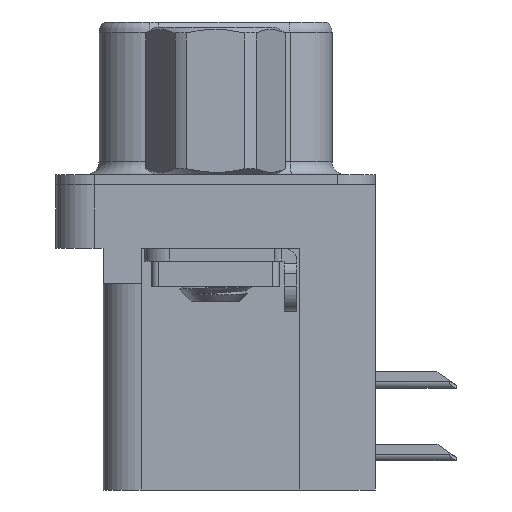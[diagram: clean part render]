
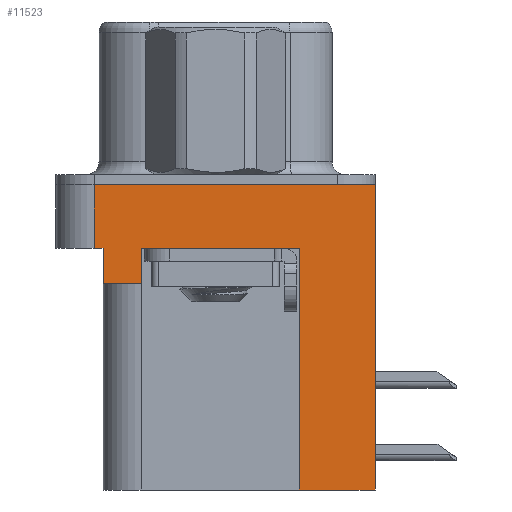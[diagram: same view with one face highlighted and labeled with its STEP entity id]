
A CAD part, left-side view. The second image highlights one B-rep face of the part: STEP entity #11523.
In plain terms, the highlighted planar face has unit normal (-1, 0, 0).
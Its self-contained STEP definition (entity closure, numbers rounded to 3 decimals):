
#674 = CARTESIAN_POINT ( 'NONE',  ( -2.91, -6.275, -2.5 ) ) ;
#1335 = VERTEX_POINT ( 'NONE', #20041 ) ;
#1969 = VECTOR ( 'NONE', #5061, 1000. ) ;
#2468 = VERTEX_POINT ( 'NONE', #5001 ) ;
#3280 = CARTESIAN_POINT ( 'NONE',  ( -2.91, -3.295, -12. ) ) ;
#3529 = VECTOR ( 'NONE', #9957, 1000. ) ;
#3999 = DIRECTION ( 'NONE',  ( 0., 1., 0. ) ) ;
#4079 = ORIENTED_EDGE ( 'NONE', *, *, #15151, .F. ) ;
#4685 = ORIENTED_EDGE ( 'NONE', *, *, #15433, .T. ) ;
#4845 = CARTESIAN_POINT ( 'NONE',  ( -2.91, 4.775, -2.5 ) ) ;
#4913 = DIRECTION ( 'NONE',  ( 0., 0., 1. ) ) ;
#4947 = ORIENTED_EDGE ( 'NONE', *, *, #13499, .T. ) ;
#5001 = CARTESIAN_POINT ( 'NONE',  ( -2.91, 4.425, -2.5 ) ) ;
#5061 = DIRECTION ( 'NONE',  ( 0., 0., 1. ) ) ;
#5863 = LINE ( 'NONE', #9686, #18467 ) ;
#6072 = VERTEX_POINT ( 'NONE', #17109 ) ;
#6803 = DIRECTION ( 'NONE',  ( 0., 1., 0. ) ) ;
#6964 = VECTOR ( 'NONE', #4913, 1000. ) ;
#7417 = ORIENTED_EDGE ( 'NONE', *, *, #13895, .T. ) ;
#7505 = VECTOR ( 'NONE', #6803, 1000. ) ;
#7864 = VERTEX_POINT ( 'NONE', #14182 ) ;
#8044 = LINE ( 'NONE', #17987, #3529 ) ;
#8852 = LINE ( 'NONE', #14051, #17487 ) ;
#9097 = VERTEX_POINT ( 'NONE', #12166 ) ;
#9280 = ORIENTED_EDGE ( 'NONE', *, *, #15211, .F. ) ;
#9686 = CARTESIAN_POINT ( 'NONE',  ( -2.91, 2.895, -3.9 ) ) ;
#9844 = CARTESIAN_POINT ( 'NONE',  ( -2.91, 4.775, 0. ) ) ;
#9957 = DIRECTION ( 'NONE',  ( 0., -1., 0. ) ) ;
#10002 = ORIENTED_EDGE ( 'NONE', *, *, #15378, .F. ) ;
#10162 = LINE ( 'NONE', #674, #11233 ) ;
#10411 = ORIENTED_EDGE ( 'NONE', *, *, #15206, .F. ) ;
#10449 = LINE ( 'NONE', #13562, #1969 ) ;
#11233 = VECTOR ( 'NONE', #12330, 1000. ) ;
#11523 = ADVANCED_FACE ( 'NONE', ( #19869 ), #17923, .T. ) ;
#11582 = DIRECTION ( 'NONE',  ( 0., 0., 1. ) ) ;
#11702 = DIRECTION ( 'NONE',  ( 0., 0., 1. ) ) ;
#11998 = LINE ( 'NONE', #4845, #16191 ) ;
#12139 = CARTESIAN_POINT ( 'NONE',  ( -2.91, -6.275, -12. ) ) ;
#12166 = CARTESIAN_POINT ( 'NONE',  ( -2.91, 2.895, -2.5 ) ) ;
#12330 = DIRECTION ( 'NONE',  ( 0., -1., 0. ) ) ;
#12501 = LINE ( 'NONE', #3280, #6964 ) ;
#12734 = CARTESIAN_POINT ( 'NONE',  ( -2.91, 4.425, -3.9 ) ) ;
#13024 = DIRECTION ( 'NONE',  ( 0., 0., 1. ) ) ;
#13079 = DIRECTION ( 'NONE',  ( 0., -1., 0. ) ) ;
#13087 = CARTESIAN_POINT ( 'NONE',  ( -2.91, -3.295, -12. ) ) ;
#13499 = EDGE_CURVE ( 'NONE', #9097, #1335, #10162, .T. ) ;
#13529 = VECTOR ( 'NONE', #13079, 1000. ) ;
#13562 = CARTESIAN_POINT ( 'NONE',  ( -2.91, -6.275, -2.5 ) ) ;
#13895 = EDGE_CURVE ( 'NONE', #6072, #9097, #5863, .T. ) ;
#14051 = CARTESIAN_POINT ( 'NONE',  ( -2.91, 4.425, -3.9 ) ) ;
#14182 = CARTESIAN_POINT ( 'NONE',  ( -2.91, 4.775, -2.5 ) ) ;
#14406 = ORIENTED_EDGE ( 'NONE', *, *, #15027, .T. ) ;
#14572 = EDGE_CURVE ( 'NONE', #6072, #20678, #8852, .T. ) ;
#14835 = DIRECTION ( 'NONE',  ( 0., 0., 1. ) ) ;
#14879 = CARTESIAN_POINT ( 'NONE',  ( -2.91, -6.275, 0. ) ) ;
#15025 = CARTESIAN_POINT ( 'NONE',  ( -2.91, -3.295, -12. ) ) ;
#15027 = EDGE_CURVE ( 'NONE', #7864, #2468, #17712, .T. ) ;
#15118 = EDGE_CURVE ( 'NONE', #18941, #16109, #8044, .T. ) ;
#15151 = EDGE_CURVE ( 'NONE', #7864, #18941, #11998, .T. ) ;
#15206 = EDGE_CURVE ( 'NONE', #20678, #2468, #19988, .T. ) ;
#15211 = EDGE_CURVE ( 'NONE', #20903, #1335, #12501, .T. ) ;
#15378 = EDGE_CURVE ( 'NONE', #15561, #20903, #18993, .T. ) ;
#15433 = EDGE_CURVE ( 'NONE', #15561, #16109, #10449, .T. ) ;
#15561 = VERTEX_POINT ( 'NONE', #12139 ) ;
#16109 = VERTEX_POINT ( 'NONE', #14879 ) ;
#16132 = CARTESIAN_POINT ( 'NONE',  ( -2.91, -6.275, -2.5 ) ) ;
#16191 = VECTOR ( 'NONE', #14835, 1000. ) ;
#16660 = ORIENTED_EDGE ( 'NONE', *, *, #14572, .F. ) ;
#16667 = ORIENTED_EDGE ( 'NONE', *, *, #15118, .F. ) ;
#17109 = CARTESIAN_POINT ( 'NONE',  ( -2.91, 2.895, -3.9 ) ) ;
#17487 = VECTOR ( 'NONE', #3999, 1000. ) ;
#17712 = LINE ( 'NONE', #16132, #13529 ) ;
#17923 = PLANE ( 'NONE',  #18416 ) ;
#17987 = CARTESIAN_POINT ( 'NONE',  ( -2.91, -6.275, 0. ) ) ;
#18402 = EDGE_LOOP ( 'NONE', ( #16667, #4079, #14406, #10411, #16660, #7417, #4947, #9280, #10002, #4685 ) ) ;
#18416 = AXIS2_PLACEMENT_3D ( 'NONE', #19562, #21103, #11582 ) ;
#18467 = VECTOR ( 'NONE', #13024, 1000. ) ;
#18941 = VERTEX_POINT ( 'NONE', #9844 ) ;
#18993 = LINE ( 'NONE', #15025, #7505 ) ;
#19562 = CARTESIAN_POINT ( 'NONE',  ( -2.91, -6.275, -2.5 ) ) ;
#19869 = FACE_OUTER_BOUND ( 'NONE', #18402, .T. ) ;
#19988 = LINE ( 'NONE', #21234, #20472 ) ;
#20041 = CARTESIAN_POINT ( 'NONE',  ( -2.91, -3.295, -2.5 ) ) ;
#20472 = VECTOR ( 'NONE', #11702, 1000. ) ;
#20678 = VERTEX_POINT ( 'NONE', #12734 ) ;
#20903 = VERTEX_POINT ( 'NONE', #13087 ) ;
#21103 = DIRECTION ( 'NONE',  ( -1., 0., 0. ) ) ;
#21234 = CARTESIAN_POINT ( 'NONE',  ( -2.91, 4.425, -3.9 ) ) ;
